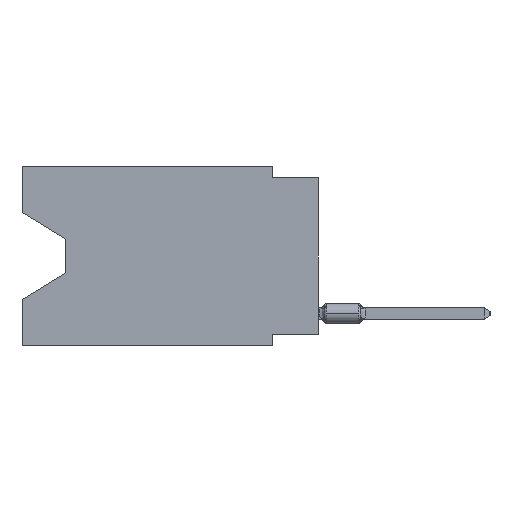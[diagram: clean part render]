
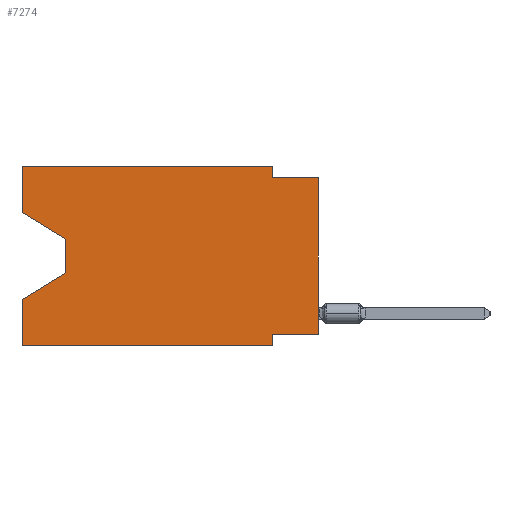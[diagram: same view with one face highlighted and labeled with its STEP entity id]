
A CAD part, left-side view. The second image highlights one B-rep face of the part: STEP entity #7274.
In plain terms, the highlighted planar face has unit normal (-1, 0, 0).
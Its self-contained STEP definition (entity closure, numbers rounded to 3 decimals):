
#606 = CARTESIAN_POINT ( 'NONE',  ( 0., 16.383, 0. ) ) ;
#689 = EDGE_CURVE ( 'NONE', #11920, #26665, #18195, .T. ) ;
#833 = LINE ( 'NONE', #9985, #8318 ) ;
#1405 = ORIENTED_EDGE ( 'NONE', *, *, #23620, .T. ) ;
#1471 = LINE ( 'NONE', #7816, #7913 ) ;
#1495 = DIRECTION ( 'NONE',  ( 0., 0., -1. ) ) ;
#1594 = DIRECTION ( 'NONE',  ( 0., 0., 1. ) ) ;
#1673 = EDGE_CURVE ( 'NONE', #27815, #4205, #833, .T. ) ;
#1818 = LINE ( 'NONE', #8308, #26294 ) ;
#2278 = CARTESIAN_POINT ( 'NONE',  ( 0., 2.54, -9.271 ) ) ;
#2673 = DIRECTION ( 'NONE',  ( 0., -1., 0. ) ) ;
#2939 = CARTESIAN_POINT ( 'NONE',  ( 0., 16.383, 0. ) ) ;
#3487 = CARTESIAN_POINT ( 'NONE',  ( 0., 16.383, -2.546 ) ) ;
#3652 = CARTESIAN_POINT ( 'NONE',  ( 0., 16.383, -9.906 ) ) ;
#3696 = VERTEX_POINT ( 'NONE', #3652 ) ;
#3821 = CARTESIAN_POINT ( 'NONE',  ( 0., 0., 0. ) ) ;
#4201 = EDGE_LOOP ( 'NONE', ( #23226, #27828, #1405, #7214, #27889, #21607, #13800, #9535, #21658, #20088, #27570, #23479 ) ) ;
#4205 = VERTEX_POINT ( 'NONE', #2278 ) ;
#4633 = VERTEX_POINT ( 'NONE', #17887 ) ;
#4865 = CARTESIAN_POINT ( 'NONE',  ( 0., 13.97, -5.893 ) ) ;
#5345 = VERTEX_POINT ( 'NONE', #17382 ) ;
#5787 = EDGE_CURVE ( 'NONE', #3696, #5345, #1818, .T. ) ;
#5793 = VERTEX_POINT ( 'NONE', #10842 ) ;
#5984 = VECTOR ( 'NONE', #22397, 1000. ) ;
#6047 = LINE ( 'NONE', #3821, #18829 ) ;
#6058 = AXIS2_PLACEMENT_3D ( 'NONE', #13883, #25254, #7659 ) ;
#6290 = VERTEX_POINT ( 'NONE', #3487 ) ;
#7214 = ORIENTED_EDGE ( 'NONE', *, *, #15605, .F. ) ;
#7274 = ADVANCED_FACE ( 'NONE', ( #25864 ), #25567, .F. ) ;
#7350 = VECTOR ( 'NONE', #25468, 1000. ) ;
#7394 = EDGE_CURVE ( 'NONE', #6290, #11920, #16252, .T. ) ;
#7659 = DIRECTION ( 'NONE',  ( 0., 0., -1. ) ) ;
#7757 = DIRECTION ( 'NONE',  ( 0., 1., 0. ) ) ;
#7816 = CARTESIAN_POINT ( 'NONE',  ( 0., 2.54, -9.906 ) ) ;
#7860 = VECTOR ( 'NONE', #28960, 1000. ) ;
#7913 = VECTOR ( 'NONE', #21872, 1000. ) ;
#8308 = CARTESIAN_POINT ( 'NONE',  ( 0., 16.383, -9.906 ) ) ;
#8318 = VECTOR ( 'NONE', #7757, 1000. ) ;
#9535 = ORIENTED_EDGE ( 'NONE', *, *, #27520, .T. ) ;
#9780 = CARTESIAN_POINT ( 'NONE',  ( 0., 16.383, -2.546 ) ) ;
#9985 = CARTESIAN_POINT ( 'NONE',  ( 0., 0., -9.271 ) ) ;
#10717 = VECTOR ( 'NONE', #1495, 1000. ) ;
#10842 = CARTESIAN_POINT ( 'NONE',  ( 0., 0., -0.635 ) ) ;
#11268 = VERTEX_POINT ( 'NONE', #17533 ) ;
#11416 = CARTESIAN_POINT ( 'NONE',  ( 0., 16.383, 0. ) ) ;
#11514 = CARTESIAN_POINT ( 'NONE',  ( 0., 16.383, -7.36 ) ) ;
#11920 = VERTEX_POINT ( 'NONE', #11416 ) ;
#12617 = VECTOR ( 'NONE', #12978, 1000. ) ;
#12745 = LINE ( 'NONE', #17754, #10717 ) ;
#12845 = LINE ( 'NONE', #14915, #12617 ) ;
#12978 = DIRECTION ( 'NONE',  ( 0., -1., 0. ) ) ;
#13800 = ORIENTED_EDGE ( 'NONE', *, *, #1673, .F. ) ;
#13883 = CARTESIAN_POINT ( 'NONE',  ( 0., 16.383, 0. ) ) ;
#14771 = DIRECTION ( 'NONE',  ( 0., 0.855, -0.519 ) ) ;
#14915 = CARTESIAN_POINT ( 'NONE',  ( 0., 0., -0.635 ) ) ;
#15188 = CARTESIAN_POINT ( 'NONE',  ( 0., 0., -9.271 ) ) ;
#15605 = EDGE_CURVE ( 'NONE', #3696, #22370, #26860, .T. ) ;
#15990 = VECTOR ( 'NONE', #16840, 1000. ) ;
#16252 = LINE ( 'NONE', #2939, #15990 ) ;
#16456 = LINE ( 'NONE', #9780, #7350 ) ;
#16840 = DIRECTION ( 'NONE',  ( 0., 0., 1. ) ) ;
#17334 = DIRECTION ( 'NONE',  ( 0., -1., 0. ) ) ;
#17382 = CARTESIAN_POINT ( 'NONE',  ( 0., 2.54, -9.906 ) ) ;
#17533 = CARTESIAN_POINT ( 'NONE',  ( 0., 2.54, -0.635 ) ) ;
#17754 = CARTESIAN_POINT ( 'NONE',  ( 0., 13.97, -4.013 ) ) ;
#17887 = CARTESIAN_POINT ( 'NONE',  ( 0., 13.97, -4.013 ) ) ;
#18195 = LINE ( 'NONE', #606, #26685 ) ;
#18829 = VECTOR ( 'NONE', #1594, 1000. ) ;
#19492 = LINE ( 'NONE', #25871, #24397 ) ;
#19638 = CARTESIAN_POINT ( 'NONE',  ( 0., 2.54, 0. ) ) ;
#20088 = ORIENTED_EDGE ( 'NONE', *, *, #23727, .F. ) ;
#20548 = EDGE_CURVE ( 'NONE', #11268, #5793, #12845, .T. ) ;
#21607 = ORIENTED_EDGE ( 'NONE', *, *, #24809, .F. ) ;
#21658 = ORIENTED_EDGE ( 'NONE', *, *, #20548, .F. ) ;
#21872 = DIRECTION ( 'NONE',  ( 0., 0., -1. ) ) ;
#22360 = CARTESIAN_POINT ( 'NONE',  ( 0., 2.54, 0. ) ) ;
#22370 = VERTEX_POINT ( 'NONE', #11514 ) ;
#22397 = DIRECTION ( 'NONE',  ( 0., 0., 1. ) ) ;
#22979 = EDGE_CURVE ( 'NONE', #6290, #4633, #16456, .T. ) ;
#23226 = ORIENTED_EDGE ( 'NONE', *, *, #22979, .T. ) ;
#23479 = ORIENTED_EDGE ( 'NONE', *, *, #7394, .F. ) ;
#23620 = EDGE_CURVE ( 'NONE', #28429, #22370, #19492, .T. ) ;
#23727 = EDGE_CURVE ( 'NONE', #26665, #11268, #28680, .T. ) ;
#24397 = VECTOR ( 'NONE', #14771, 1000. ) ;
#24750 = CARTESIAN_POINT ( 'NONE',  ( 0., 16.383, 0. ) ) ;
#24809 = EDGE_CURVE ( 'NONE', #4205, #5345, #1471, .T. ) ;
#25254 = DIRECTION ( 'NONE',  ( 1., 0., 0. ) ) ;
#25468 = DIRECTION ( 'NONE',  ( 0., -0.855, -0.519 ) ) ;
#25567 = PLANE ( 'NONE',  #6058 ) ;
#25864 = FACE_OUTER_BOUND ( 'NONE', #4201, .T. ) ;
#25871 = CARTESIAN_POINT ( 'NONE',  ( 0., 13.97, -5.893 ) ) ;
#26294 = VECTOR ( 'NONE', #17334, 1000. ) ;
#26665 = VERTEX_POINT ( 'NONE', #22360 ) ;
#26685 = VECTOR ( 'NONE', #2673, 1000. ) ;
#26860 = LINE ( 'NONE', #24750, #5984 ) ;
#27520 = EDGE_CURVE ( 'NONE', #27815, #5793, #6047, .T. ) ;
#27570 = ORIENTED_EDGE ( 'NONE', *, *, #689, .F. ) ;
#27815 = VERTEX_POINT ( 'NONE', #15188 ) ;
#27828 = ORIENTED_EDGE ( 'NONE', *, *, #28324, .T. ) ;
#27889 = ORIENTED_EDGE ( 'NONE', *, *, #5787, .T. ) ;
#28324 = EDGE_CURVE ( 'NONE', #4633, #28429, #12745, .T. ) ;
#28429 = VERTEX_POINT ( 'NONE', #4865 ) ;
#28680 = LINE ( 'NONE', #19638, #7860 ) ;
#28960 = DIRECTION ( 'NONE',  ( 0., 0., -1. ) ) ;
